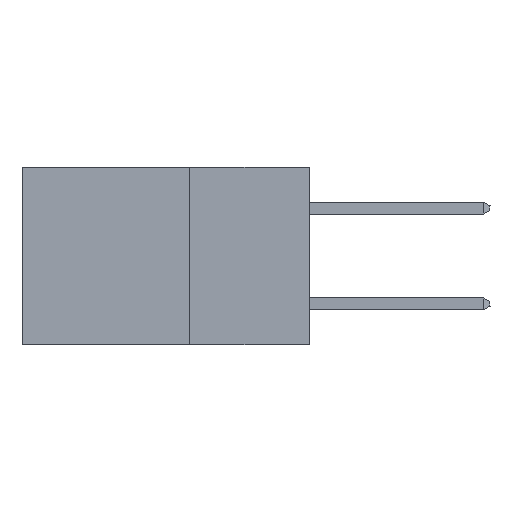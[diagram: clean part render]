
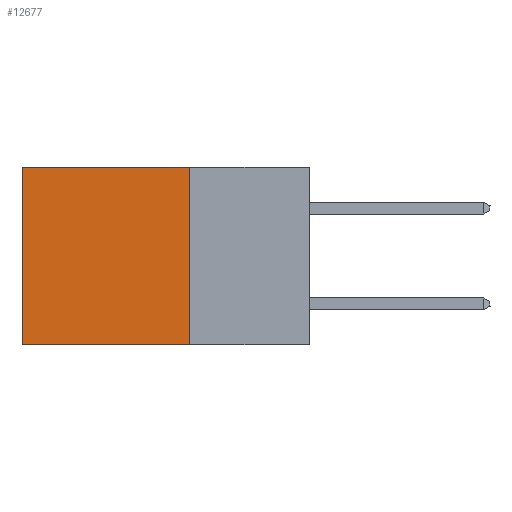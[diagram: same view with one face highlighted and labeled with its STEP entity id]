
A CAD part, left-side view. The second image highlights one B-rep face of the part: STEP entity #12677.
In plain terms, the highlighted planar face has unit normal (-1, 0, 0).
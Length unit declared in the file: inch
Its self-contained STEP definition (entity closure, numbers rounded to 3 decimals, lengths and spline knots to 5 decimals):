
#533 = VECTOR ( 'NONE', #19205, 39.37008 ) ;
#803 = EDGE_CURVE ( 'NONE', #39932, #7761, #15347, .T. ) ;
#2281 = ORIENTED_EDGE ( 'NONE', *, *, #29231, .F. ) ;
#3612 = EDGE_LOOP ( 'NONE', ( #30855, #24380, #2281, #6565 ) ) ;
#4474 = CARTESIAN_POINT ( 'NONE',  ( 0.2875, 0.6, -0.37 ) ) ;
#6565 = ORIENTED_EDGE ( 'NONE', *, *, #28717, .T. ) ;
#6895 = VECTOR ( 'NONE', #39802, 39.37008 ) ;
#7761 = VERTEX_POINT ( 'NONE', #4474 ) ;
#9717 = CARTESIAN_POINT ( 'NONE',  ( 0.2875, 0.6, 0. ) ) ;
#10376 = CARTESIAN_POINT ( 'NONE',  ( 0.2875, 0.25, 0. ) ) ;
#12079 = VECTOR ( 'NONE', #13685, 39.37008 ) ;
#12677 = ADVANCED_FACE ( 'NONE', ( #17800 ), #32380, .F. ) ;
#13685 = DIRECTION ( 'NONE',  ( 0., 1., 0. ) ) ;
#14413 = LINE ( 'NONE', #15072, #21836 ) ;
#15072 = CARTESIAN_POINT ( 'NONE',  ( 0.2875, 0.25, -0.37 ) ) ;
#15347 = LINE ( 'NONE', #30506, #6895 ) ;
#15941 = AXIS2_PLACEMENT_3D ( 'NONE', #26195, #16905, #38583 ) ;
#16049 = CARTESIAN_POINT ( 'NONE',  ( 0.2875, 0.25, 0. ) ) ;
#16905 = DIRECTION ( 'NONE',  ( 1., 0., 0. ) ) ;
#17800 = FACE_OUTER_BOUND ( 'NONE', #3612, .T. ) ;
#19205 = DIRECTION ( 'NONE',  ( 0., 0., -1. ) ) ;
#21418 = DIRECTION ( 'NONE',  ( 0., 1., 0. ) ) ;
#21836 = VECTOR ( 'NONE', #21418, 39.37008 ) ;
#24380 = ORIENTED_EDGE ( 'NONE', *, *, #35739, .F. ) ;
#26195 = CARTESIAN_POINT ( 'NONE',  ( 0.2875, 0.25, 0. ) ) ;
#26215 = CARTESIAN_POINT ( 'NONE',  ( 0.2875, 0.25, 0. ) ) ;
#26861 = LINE ( 'NONE', #16049, #533 ) ;
#28195 = VERTEX_POINT ( 'NONE', #10376 ) ;
#28717 = EDGE_CURVE ( 'NONE', #28195, #39932, #37011, .T. ) ;
#29231 = EDGE_CURVE ( 'NONE', #28195, #30575, #26861, .T. ) ;
#30506 = CARTESIAN_POINT ( 'NONE',  ( 0.2875, 0.6, 0. ) ) ;
#30575 = VERTEX_POINT ( 'NONE', #31456 ) ;
#30855 = ORIENTED_EDGE ( 'NONE', *, *, #803, .T. ) ;
#31456 = CARTESIAN_POINT ( 'NONE',  ( 0.2875, 0.25, -0.37 ) ) ;
#32380 = PLANE ( 'NONE',  #15941 ) ;
#35739 = EDGE_CURVE ( 'NONE', #30575, #7761, #14413, .T. ) ;
#37011 = LINE ( 'NONE', #26215, #12079 ) ;
#38583 = DIRECTION ( 'NONE',  ( 0., 0., -1. ) ) ;
#39802 = DIRECTION ( 'NONE',  ( 0., 0., -1. ) ) ;
#39932 = VERTEX_POINT ( 'NONE', #9717 ) ;
